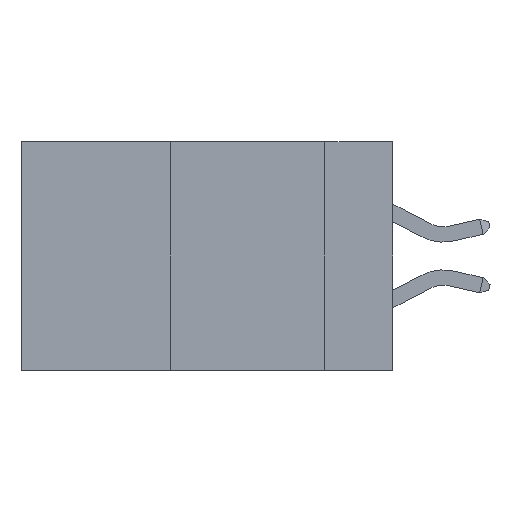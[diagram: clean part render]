
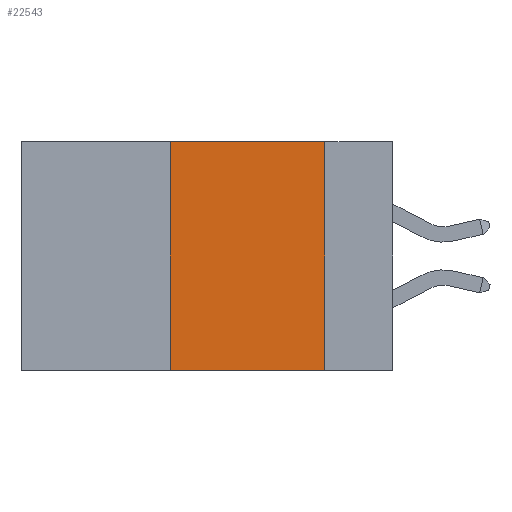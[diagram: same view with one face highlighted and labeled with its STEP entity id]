
A CAD part, left-side view. The second image highlights one B-rep face of the part: STEP entity #22543.
In plain terms, the highlighted planar face has unit normal (-1, 0, 0).
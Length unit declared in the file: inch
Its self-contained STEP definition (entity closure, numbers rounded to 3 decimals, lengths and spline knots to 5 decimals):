
#556 = ORIENTED_EDGE ( 'NONE', *, *, #27641, .F. ) ;
#569 = CARTESIAN_POINT ( 'NONE',  ( 0., 0.36, -0.37 ) ) ;
#3064 = AXIS2_PLACEMENT_3D ( 'NONE', #29453, #29350, #14638 ) ;
#4469 = VECTOR ( 'NONE', #6956, 39.37008 ) ;
#5432 = CARTESIAN_POINT ( 'NONE',  ( 0., 0.11, 0. ) ) ;
#6738 = CARTESIAN_POINT ( 'NONE',  ( 0., 0.6, 0. ) ) ;
#6907 = ORIENTED_EDGE ( 'NONE', *, *, #14335, .F. ) ;
#6956 = DIRECTION ( 'NONE',  ( 0., -1., 0. ) ) ;
#7371 = LINE ( 'NONE', #27355, #7724 ) ;
#7724 = VECTOR ( 'NONE', #15994, 39.37008 ) ;
#7779 = VERTEX_POINT ( 'NONE', #8221 ) ;
#7913 = VERTEX_POINT ( 'NONE', #569 ) ;
#8221 = CARTESIAN_POINT ( 'NONE',  ( 0., 0.11, -0.37 ) ) ;
#9119 = EDGE_CURVE ( 'NONE', #7913, #7779, #20686, .T. ) ;
#9653 = VECTOR ( 'NONE', #27982, 39.37008 ) ;
#10376 = EDGE_LOOP ( 'NONE', ( #6907, #31736, #556, #12257 ) ) ;
#12173 = PLANE ( 'NONE',  #3064 ) ;
#12257 = ORIENTED_EDGE ( 'NONE', *, *, #9119, .T. ) ;
#13637 = CARTESIAN_POINT ( 'NONE',  ( 0., 0.11, 0. ) ) ;
#14162 = LINE ( 'NONE', #6738, #4469 ) ;
#14335 = EDGE_CURVE ( 'NONE', #29587, #7779, #16176, .T. ) ;
#14638 = DIRECTION ( 'NONE',  ( 0., 0., -1. ) ) ;
#15994 = DIRECTION ( 'NONE',  ( 0., 0., 1. ) ) ;
#16176 = LINE ( 'NONE', #13637, #9653 ) ;
#16985 = CARTESIAN_POINT ( 'NONE',  ( 0., 0.6, -0.37 ) ) ;
#20575 = CARTESIAN_POINT ( 'NONE',  ( 0., 0.36, 0. ) ) ;
#20686 = LINE ( 'NONE', #16985, #24224 ) ;
#22543 = ADVANCED_FACE ( 'NONE', ( #31603 ), #12173, .F. ) ;
#23844 = EDGE_CURVE ( 'NONE', #26030, #29587, #14162, .T. ) ;
#24224 = VECTOR ( 'NONE', #26747, 39.37008 ) ;
#26030 = VERTEX_POINT ( 'NONE', #20575 ) ;
#26747 = DIRECTION ( 'NONE',  ( 0., -1., 0. ) ) ;
#27355 = CARTESIAN_POINT ( 'NONE',  ( 0., 0.36, 0. ) ) ;
#27641 = EDGE_CURVE ( 'NONE', #7913, #26030, #7371, .T. ) ;
#27982 = DIRECTION ( 'NONE',  ( 0., 0., -1. ) ) ;
#29350 = DIRECTION ( 'NONE',  ( 1., 0., 0. ) ) ;
#29453 = CARTESIAN_POINT ( 'NONE',  ( 0., 0.6, 0. ) ) ;
#29587 = VERTEX_POINT ( 'NONE', #5432 ) ;
#31603 = FACE_OUTER_BOUND ( 'NONE', #10376, .T. ) ;
#31736 = ORIENTED_EDGE ( 'NONE', *, *, #23844, .F. ) ;
